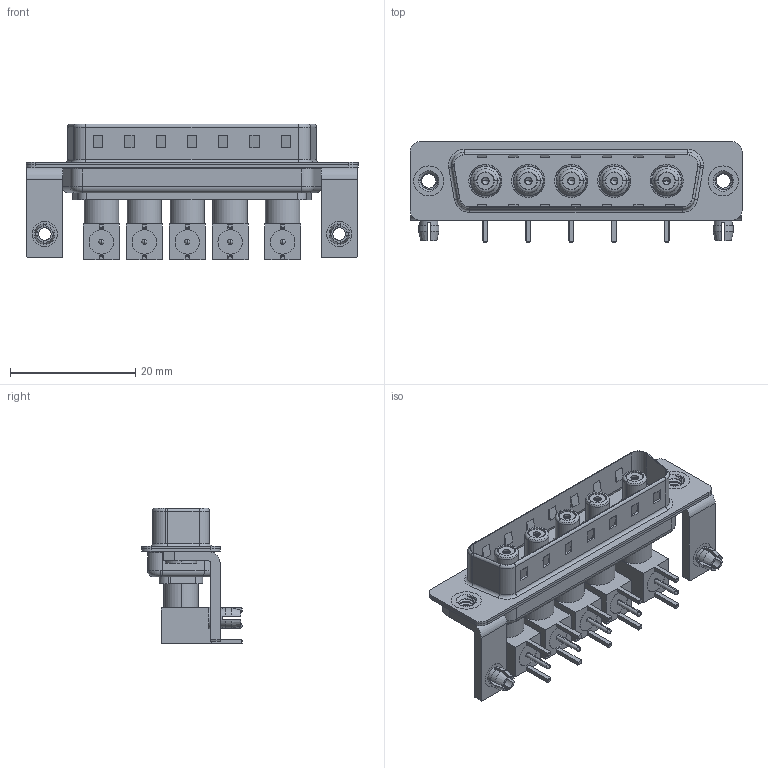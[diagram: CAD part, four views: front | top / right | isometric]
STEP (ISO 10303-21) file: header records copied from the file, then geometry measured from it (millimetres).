
FILE_DESCRIPTION (( 'STEP AP203' ), '1' );
FILE_NAME ('629-5W5-240-7N3.STEP', '2022-05-07T06:04:05', ( '' ), ( '' ), 'SwSTEP 2.0', 'SolidWorks 2020', '' );
FILE_SCHEMA (( 'CONFIG_CONTROL_DESIGN' ));
Length unit declared in the file: millimetre
Products named in the file (19): 629Combo Threaded Rivet_3; 629Combo Housing_5W5; Insulator Socket; 629Combo Board Lock; Insulator RA Pin; Co-Ax Jack Assy_RA; Socket_RA; 629Combo Stabilizer Bracket; 629-5W5-240-7N3; Locking Collar; Co-Ax Jack_RA PC Tail; 629Combo Shell Front_25 Contacts; Insulator Socket 2; RA Back Shell; 629Combo Shell Rear_25 Contacts
Assembly tree (49 placements, depth 3):
  629-5W5-240-7N3
    629Combo Housing_5W5
    629Combo Shell Rear_25 Contacts
    629Combo Shell Front_25 Contacts
    629Combo Threaded Rivet_3  x2
    629Combo Stabilizer Bracket  x2
    629Combo Board Lock  x2
    Co-Ax Jack Assy_RA
      Co-Ax Jack_RA PC Tail
      Insulator Socket
      Insulator Socket 2
      Locking Collar
      Socket_RA
      RA Back Shell
      Insulator RA Pin
    Co-Ax Jack Assy_RA
      Co-Ax Jack_RA PC Tail
      Insulator Socket
      Insulator Socket 2
      Locking Collar
      Socket_RA
      RA Back Shell
      Insulator RA Pin
    Co-Ax Jack Assy_RA
      Co-Ax Jack_RA PC Tail
      Insulator Socket
      Insulator Socket 2
      Locking Collar
      Socket_RA
      RA Back Shell
      Insulator RA Pin
    Co-Ax Jack Assy_RA
      Co-Ax Jack_RA PC Tail
      Insulator Socket
      Insulator Socket 2
      Locking Collar
      Socket_RA
      RA Back Shell
      Insulator RA Pin
    Co-Ax Jack Assy_RA
      Co-Ax Jack_RA PC Tail
      Insulator Socket
      Insulator Socket 2
      Locking Collar
      Socket_RA
      RA Back Shell
      Insulator RA Pin
Bounding box: 53.05 x 16 x 21.71 mm (x, y, z)
Volume: 4447.4 mm3; surface area: 12165.9 mm2
Topology: 44 solids, 44 shells, 1268 faces, 3032 edges, 1897 vertices
Faces by surface type: plane 524, cylinder 522, cone 121, torus 80, bspline 11, sphere 10
Entity records: 21908 total; most frequent: CARTESIAN_POINT 4689, DIRECTION 3192, ORIENTED_EDGE 2864, EDGE_CURVE 1432, AXIS2_PLACEMENT_3D 1193, VERTEX_POINT 908, VECTOR 806, LINE 806
